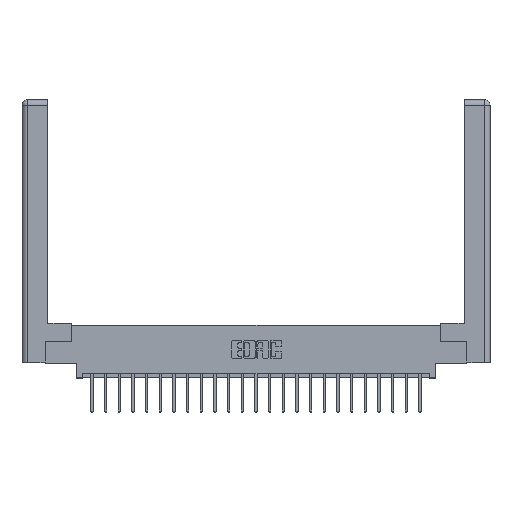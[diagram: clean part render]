
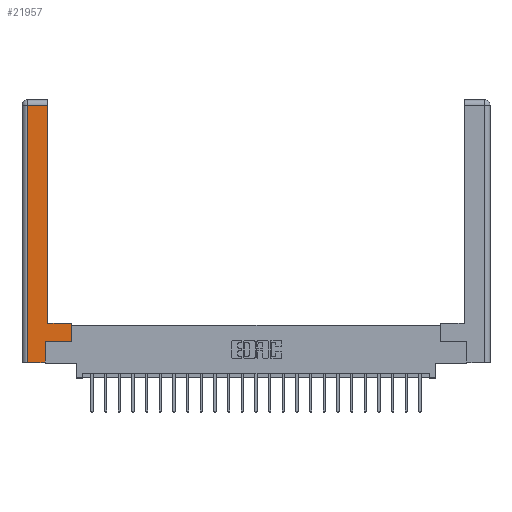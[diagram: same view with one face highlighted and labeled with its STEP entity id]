
A CAD part, top view. The second image highlights one B-rep face of the part: STEP entity #21957.
In plain terms, the highlighted planar face has unit normal (0, 0, 1).
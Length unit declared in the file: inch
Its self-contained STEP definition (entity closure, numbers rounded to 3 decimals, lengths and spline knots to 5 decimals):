
#1205 = EDGE_CURVE ( 'NONE', #20945, #22739, #9613, .T. ) ;
#1306 = EDGE_LOOP ( 'NONE', ( #15142, #19542, #6272, #13252, #13226, #9956, #14554, #22306 ) ) ;
#1529 = AXIS2_PLACEMENT_3D ( 'NONE', #22926, #16368, #12522 ) ;
#1892 = DIRECTION ( 'NONE',  ( -1., 0., 0. ) ) ;
#2084 = EDGE_CURVE ( 'NONE', #18614, #22023, #10496, .T. ) ;
#2939 = VECTOR ( 'NONE', #7792, 39.37008 ) ;
#3081 = CARTESIAN_POINT ( 'NONE',  ( 0.565, 0.245, 0. ) ) ;
#3198 = DIRECTION ( 'NONE',  ( 0., 1., 0. ) ) ;
#3211 = CARTESIAN_POINT ( 'NONE',  ( 0.565, 0.45, 0. ) ) ;
#3234 = VECTOR ( 'NONE', #17898, 39.37008 ) ;
#3479 = CARTESIAN_POINT ( 'NONE',  ( 0.565, 0.45, 0. ) ) ;
#3835 = LINE ( 'NONE', #8025, #3234 ) ;
#4030 = CARTESIAN_POINT ( 'NONE',  ( 0.265, 0.245, 0. ) ) ;
#4815 = CARTESIAN_POINT ( 'NONE',  ( 0.265, 0., 0. ) ) ;
#5196 = VECTOR ( 'NONE', #7259, 39.37008 ) ;
#5482 = VECTOR ( 'NONE', #22101, 39.37008 ) ;
#5545 = LINE ( 'NONE', #6999, #8754 ) ;
#6272 = ORIENTED_EDGE ( 'NONE', *, *, #14241, .T. ) ;
#6999 = CARTESIAN_POINT ( 'NONE',  ( 0.0615, 0., 0. ) ) ;
#7259 = DIRECTION ( 'NONE',  ( 1., 0., 0. ) ) ;
#7356 = CARTESIAN_POINT ( 'NONE',  ( 0.265, 0., 0. ) ) ;
#7792 = DIRECTION ( 'NONE',  ( -1., 0., 0. ) ) ;
#8010 = PLANE ( 'NONE',  #1529 ) ;
#8025 = CARTESIAN_POINT ( 'NONE',  ( 0.565, 0.245, 0. ) ) ;
#8273 = LINE ( 'NONE', #13169, #15645 ) ;
#8628 = CARTESIAN_POINT ( 'NONE',  ( 0.295, 2.94, 0. ) ) ;
#8754 = VECTOR ( 'NONE', #16446, 39.37008 ) ;
#8926 = EDGE_CURVE ( 'NONE', #9847, #22002, #23756, .T. ) ;
#9613 = LINE ( 'NONE', #19227, #19059 ) ;
#9847 = VERTEX_POINT ( 'NONE', #15463 ) ;
#9956 = ORIENTED_EDGE ( 'NONE', *, *, #13277, .T. ) ;
#9963 = VERTEX_POINT ( 'NONE', #4030 ) ;
#10437 = CARTESIAN_POINT ( 'NONE',  ( 0.265, 0.245, 0. ) ) ;
#10496 = LINE ( 'NONE', #3479, #5482 ) ;
#10518 = FACE_OUTER_BOUND ( 'NONE', #1306, .T. ) ;
#11793 = EDGE_CURVE ( 'NONE', #22739, #23352, #8273, .T. ) ;
#12473 = CARTESIAN_POINT ( 'NONE',  ( 0.0615, 2.94, 0. ) ) ;
#12522 = DIRECTION ( 'NONE',  ( -1., 0., 0. ) ) ;
#13117 = EDGE_CURVE ( 'NONE', #22023, #20945, #17680, .T. ) ;
#13169 = CARTESIAN_POINT ( 'NONE',  ( 0.0615, 2.94, 0. ) ) ;
#13226 = ORIENTED_EDGE ( 'NONE', *, *, #15170, .T. ) ;
#13252 = ORIENTED_EDGE ( 'NONE', *, *, #8926, .T. ) ;
#13277 = EDGE_CURVE ( 'NONE', #9963, #18614, #3835, .T. ) ;
#14241 = EDGE_CURVE ( 'NONE', #23352, #9847, #5545, .T. ) ;
#14554 = ORIENTED_EDGE ( 'NONE', *, *, #2084, .T. ) ;
#15142 = ORIENTED_EDGE ( 'NONE', *, *, #1205, .T. ) ;
#15170 = EDGE_CURVE ( 'NONE', #22002, #9963, #19555, .T. ) ;
#15463 = CARTESIAN_POINT ( 'NONE',  ( 0.0615, 0., 0. ) ) ;
#15645 = VECTOR ( 'NONE', #1892, 39.37008 ) ;
#16368 = DIRECTION ( 'NONE',  ( 0., 0., -1. ) ) ;
#16446 = DIRECTION ( 'NONE',  ( 0., -1., 0. ) ) ;
#17680 = LINE ( 'NONE', #19078, #2939 ) ;
#17898 = DIRECTION ( 'NONE',  ( 1., 0., 0. ) ) ;
#18614 = VERTEX_POINT ( 'NONE', #3081 ) ;
#18970 = VECTOR ( 'NONE', #23581, 39.37008 ) ;
#19059 = VECTOR ( 'NONE', #3198, 39.37008 ) ;
#19078 = CARTESIAN_POINT ( 'NONE',  ( 0.295, 0.45, 0. ) ) ;
#19227 = CARTESIAN_POINT ( 'NONE',  ( 0.295, 3., 0. ) ) ;
#19542 = ORIENTED_EDGE ( 'NONE', *, *, #11793, .T. ) ;
#19555 = LINE ( 'NONE', #10437, #18970 ) ;
#20945 = VERTEX_POINT ( 'NONE', #23031 ) ;
#21957 = ADVANCED_FACE ( 'NONE', ( #10518 ), #8010, .F. ) ;
#22002 = VERTEX_POINT ( 'NONE', #4815 ) ;
#22023 = VERTEX_POINT ( 'NONE', #3211 ) ;
#22101 = DIRECTION ( 'NONE',  ( 0., 1., 0. ) ) ;
#22306 = ORIENTED_EDGE ( 'NONE', *, *, #13117, .T. ) ;
#22739 = VERTEX_POINT ( 'NONE', #8628 ) ;
#22926 = CARTESIAN_POINT ( 'NONE',  ( 0., 0., 0. ) ) ;
#23031 = CARTESIAN_POINT ( 'NONE',  ( 0.295, 0.45, 0. ) ) ;
#23352 = VERTEX_POINT ( 'NONE', #12473 ) ;
#23581 = DIRECTION ( 'NONE',  ( 0., 1., 0. ) ) ;
#23756 = LINE ( 'NONE', #7356, #5196 ) ;
